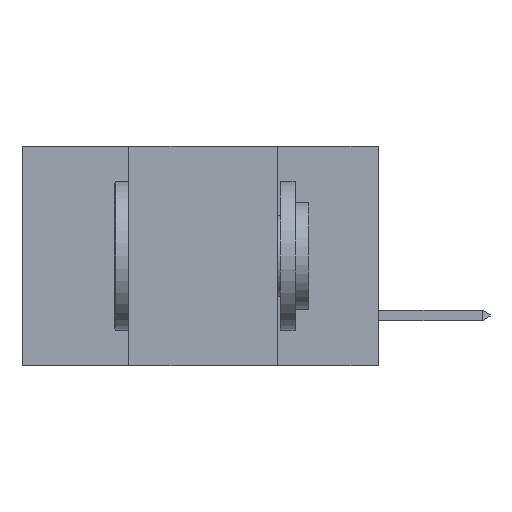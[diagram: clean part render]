
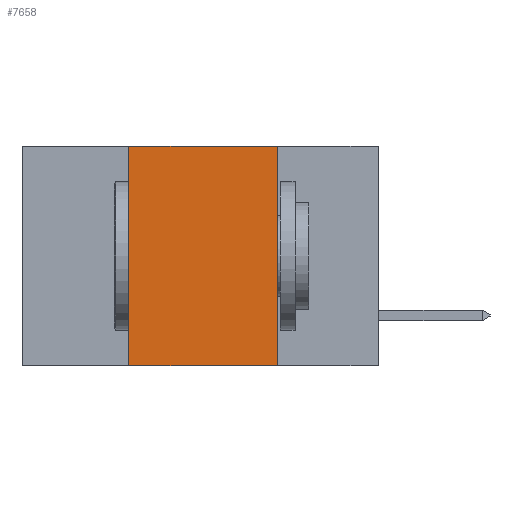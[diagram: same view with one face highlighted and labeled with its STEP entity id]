
A CAD part, left-side view. The second image highlights one B-rep face of the part: STEP entity #7658.
In plain terms, the highlighted planar face has unit normal (-1, 0, 0).
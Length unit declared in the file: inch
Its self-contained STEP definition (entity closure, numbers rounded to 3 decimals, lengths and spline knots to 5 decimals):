
#664 = DIRECTION ( 'NONE',  ( 0., -1., 0. ) ) ;
#771 = VECTOR ( 'NONE', #664, 39.37008 ) ;
#1213 = DIRECTION ( 'NONE',  ( 0., 0., -1. ) ) ;
#2290 = FACE_OUTER_BOUND ( 'NONE', #9337, .T. ) ;
#2398 = VECTOR ( 'NONE', #17395, 39.37008 ) ;
#3036 = VERTEX_POINT ( 'NONE', #13951 ) ;
#3389 = VERTEX_POINT ( 'NONE', #8842 ) ;
#3747 = ORIENTED_EDGE ( 'NONE', *, *, #16680, .F. ) ;
#4573 = DIRECTION ( 'NONE',  ( 0., -1., 0. ) ) ;
#5247 = AXIS2_PLACEMENT_3D ( 'NONE', #16510, #9595, #1213 ) ;
#5862 = CARTESIAN_POINT ( 'NONE',  ( 0., 0.17, 0. ) ) ;
#5929 = LINE ( 'NONE', #15259, #9638 ) ;
#6930 = DIRECTION ( 'NONE',  ( 0., 0., -1. ) ) ;
#7658 = ADVANCED_FACE ( 'NONE', ( #2290 ), #17900, .F. ) ;
#7984 = CARTESIAN_POINT ( 'NONE',  ( 0., 0.42, -0.37 ) ) ;
#8842 = CARTESIAN_POINT ( 'NONE',  ( 0., 0.42, 0. ) ) ;
#9337 = EDGE_LOOP ( 'NONE', ( #10763, #3747, #12699, #11190 ) ) ;
#9595 = DIRECTION ( 'NONE',  ( 1., 0., 0. ) ) ;
#9638 = VECTOR ( 'NONE', #6930, 39.37008 ) ;
#9778 = EDGE_CURVE ( 'NONE', #15310, #3036, #5929, .T. ) ;
#10763 = ORIENTED_EDGE ( 'NONE', *, *, #9778, .F. ) ;
#11190 = ORIENTED_EDGE ( 'NONE', *, *, #14971, .T. ) ;
#11816 = EDGE_CURVE ( 'NONE', #11986, #3389, #13539, .T. ) ;
#11867 = CARTESIAN_POINT ( 'NONE',  ( 0., 0.42, 0. ) ) ;
#11986 = VERTEX_POINT ( 'NONE', #7984 ) ;
#12699 = ORIENTED_EDGE ( 'NONE', *, *, #11816, .F. ) ;
#13260 = CARTESIAN_POINT ( 'NONE',  ( 0., 0.6, -0.37 ) ) ;
#13539 = LINE ( 'NONE', #11867, #2398 ) ;
#13795 = LINE ( 'NONE', #14332, #17482 ) ;
#13951 = CARTESIAN_POINT ( 'NONE',  ( 0., 0.17, -0.37 ) ) ;
#14332 = CARTESIAN_POINT ( 'NONE',  ( 0., 0.6, 0. ) ) ;
#14729 = LINE ( 'NONE', #13260, #771 ) ;
#14971 = EDGE_CURVE ( 'NONE', #11986, #3036, #14729, .T. ) ;
#15259 = CARTESIAN_POINT ( 'NONE',  ( 0., 0.17, 0. ) ) ;
#15310 = VERTEX_POINT ( 'NONE', #5862 ) ;
#16510 = CARTESIAN_POINT ( 'NONE',  ( 0., 0.6, 0. ) ) ;
#16680 = EDGE_CURVE ( 'NONE', #3389, #15310, #13795, .T. ) ;
#17395 = DIRECTION ( 'NONE',  ( 0., 0., 1. ) ) ;
#17482 = VECTOR ( 'NONE', #4573, 39.37008 ) ;
#17900 = PLANE ( 'NONE',  #5247 ) ;
